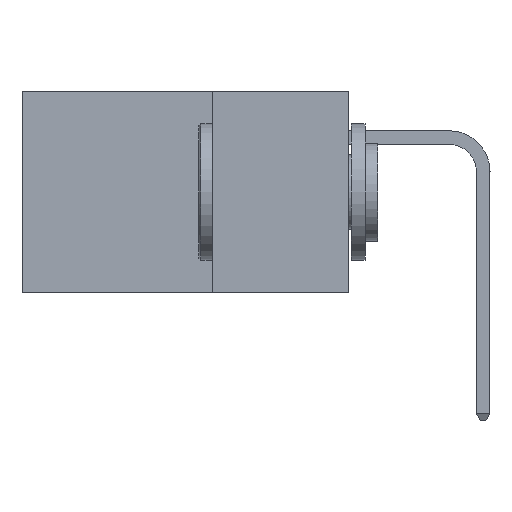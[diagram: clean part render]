
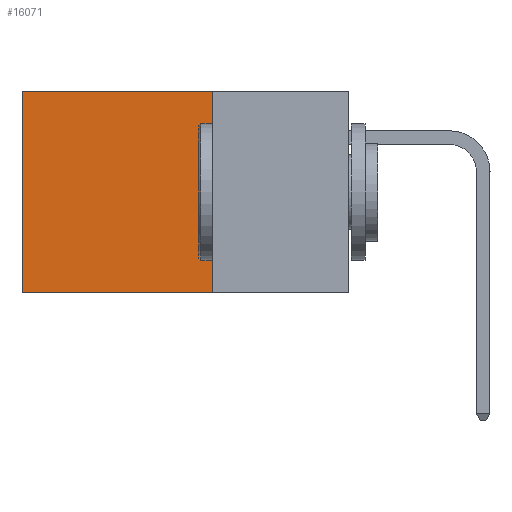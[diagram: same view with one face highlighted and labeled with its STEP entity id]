
A CAD part, left-side view. The second image highlights one B-rep face of the part: STEP entity #16071.
In plain terms, the highlighted planar face has unit normal (-1, 0, 0).
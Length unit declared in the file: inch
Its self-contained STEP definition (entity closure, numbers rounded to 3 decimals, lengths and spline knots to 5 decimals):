
#225 = VECTOR ( 'NONE', #22906, 39.37008 ) ;
#529 = CARTESIAN_POINT ( 'NONE',  ( 0.2875, 0.25, -0.37 ) ) ;
#1184 = AXIS2_PLACEMENT_3D ( 'NONE', #31461, #38876, #28838 ) ;
#2634 = EDGE_CURVE ( 'NONE', #9771, #9870, #2677, .T. ) ;
#2677 = LINE ( 'NONE', #23123, #16890 ) ;
#3646 = ORIENTED_EDGE ( 'NONE', *, *, #35608, .F. ) ;
#3696 = EDGE_CURVE ( 'NONE', #9771, #17963, #25546, .T. ) ;
#6981 = LINE ( 'NONE', #529, #40583 ) ;
#7538 = ORIENTED_EDGE ( 'NONE', *, *, #3696, .F. ) ;
#9771 = VERTEX_POINT ( 'NONE', #40936 ) ;
#9870 = VERTEX_POINT ( 'NONE', #15906 ) ;
#10564 = DIRECTION ( 'NONE',  ( 0., 1., 0. ) ) ;
#12130 = ORIENTED_EDGE ( 'NONE', *, *, #2634, .T. ) ;
#12617 = CARTESIAN_POINT ( 'NONE',  ( 0.2875, 0.6, -0.37 ) ) ;
#13758 = CARTESIAN_POINT ( 'NONE',  ( 0.2875, 0.25, 0. ) ) ;
#13841 = VECTOR ( 'NONE', #23136, 39.37008 ) ;
#15906 = CARTESIAN_POINT ( 'NONE',  ( 0.2875, 0.6, 0. ) ) ;
#16071 = ADVANCED_FACE ( 'NONE', ( #21475 ), #27739, .F. ) ;
#16624 = CARTESIAN_POINT ( 'NONE',  ( 0.2875, 0.6, 0. ) ) ;
#16890 = VECTOR ( 'NONE', #16985, 39.37008 ) ;
#16985 = DIRECTION ( 'NONE',  ( 0., 1., 0. ) ) ;
#17963 = VERTEX_POINT ( 'NONE', #29218 ) ;
#21475 = FACE_OUTER_BOUND ( 'NONE', #28871, .T. ) ;
#22906 = DIRECTION ( 'NONE',  ( 0., 0., -1. ) ) ;
#23123 = CARTESIAN_POINT ( 'NONE',  ( 0.2875, 0.25, 0. ) ) ;
#23136 = DIRECTION ( 'NONE',  ( 0., 0., -1. ) ) ;
#25546 = LINE ( 'NONE', #13758, #13841 ) ;
#27739 = PLANE ( 'NONE',  #1184 ) ;
#27751 = LINE ( 'NONE', #16624, #225 ) ;
#28838 = DIRECTION ( 'NONE',  ( 0., 0., -1. ) ) ;
#28871 = EDGE_LOOP ( 'NONE', ( #35438, #3646, #7538, #12130 ) ) ;
#29218 = CARTESIAN_POINT ( 'NONE',  ( 0.2875, 0.25, -0.37 ) ) ;
#29500 = EDGE_CURVE ( 'NONE', #9870, #39339, #27751, .T. ) ;
#31461 = CARTESIAN_POINT ( 'NONE',  ( 0.2875, 0.25, 0. ) ) ;
#35438 = ORIENTED_EDGE ( 'NONE', *, *, #29500, .T. ) ;
#35608 = EDGE_CURVE ( 'NONE', #17963, #39339, #6981, .T. ) ;
#38876 = DIRECTION ( 'NONE',  ( 1., 0., 0. ) ) ;
#39339 = VERTEX_POINT ( 'NONE', #12617 ) ;
#40583 = VECTOR ( 'NONE', #10564, 39.37008 ) ;
#40936 = CARTESIAN_POINT ( 'NONE',  ( 0.2875, 0.25, 0. ) ) ;
